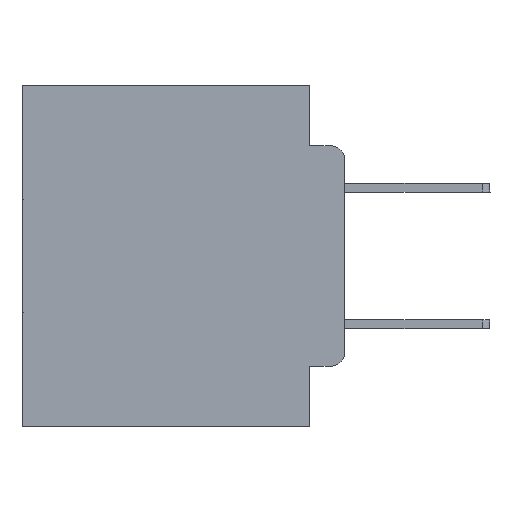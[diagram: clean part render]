
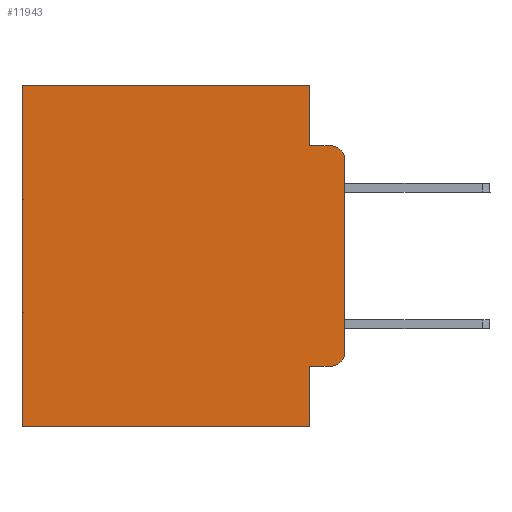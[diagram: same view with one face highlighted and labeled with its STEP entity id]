
A CAD part, left-side view. The second image highlights one B-rep face of the part: STEP entity #11943.
In plain terms, the highlighted planar face has unit normal (-1, 0, 0).
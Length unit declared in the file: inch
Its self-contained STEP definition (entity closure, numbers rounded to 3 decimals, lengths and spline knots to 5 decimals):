
#215 = VERTEX_POINT ( 'NONE', #12271 ) ;
#527 = DIRECTION ( 'NONE',  ( -1., 0., 0. ) ) ;
#592 = VECTOR ( 'NONE', #7287, 39.37008 ) ;
#806 = PLANE ( 'NONE',  #26116 ) ;
#974 = VECTOR ( 'NONE', #10853, 39.37008 ) ;
#2028 = EDGE_CURVE ( 'NONE', #20174, #215, #22887, .T. ) ;
#2127 = VERTEX_POINT ( 'NONE', #13937 ) ;
#3052 = CARTESIAN_POINT ( 'NONE',  ( 0.298, 0.051, 0. ) ) ;
#3873 = EDGE_CURVE ( 'NONE', #20174, #5338, #8511, .T. ) ;
#3918 = VECTOR ( 'NONE', #6177, 39.37008 ) ;
#4004 = CIRCLE ( 'NONE', #19511, 0.02 ) ;
#4091 = VERTEX_POINT ( 'NONE', #21742 ) ;
#4457 = VERTEX_POINT ( 'NONE', #24705 ) ;
#5199 = CARTESIAN_POINT ( 'NONE',  ( 0.298, 0., 0. ) ) ;
#5338 = VERTEX_POINT ( 'NONE', #29000 ) ;
#5693 = DIRECTION ( 'NONE',  ( 0., 0., -1. ) ) ;
#5732 = ORIENTED_EDGE ( 'NONE', *, *, #3873, .F. ) ;
#5999 = LINE ( 'NONE', #8336, #18496 ) ;
#6177 = DIRECTION ( 'NONE',  ( 0., 0., -1. ) ) ;
#6670 = VECTOR ( 'NONE', #21443, 39.37008 ) ;
#7141 = CARTESIAN_POINT ( 'NONE',  ( 0.298, 0.051, -0.4115 ) ) ;
#7287 = DIRECTION ( 'NONE',  ( 0., -1., 0. ) ) ;
#7896 = LINE ( 'NONE', #27117, #17403 ) ;
#8109 = CARTESIAN_POINT ( 'NONE',  ( 0.298, 0.051, -0.0885 ) ) ;
#8336 = CARTESIAN_POINT ( 'NONE',  ( 0.298, 0., -0.5 ) ) ;
#8511 = LINE ( 'NONE', #3052, #3918 ) ;
#8610 = EDGE_CURVE ( 'NONE', #11985, #4457, #7896, .T. ) ;
#8725 = EDGE_CURVE ( 'NONE', #215, #26105, #4004, .T. ) ;
#9983 = EDGE_CURVE ( 'NONE', #30833, #4091, #23713, .T. ) ;
#10091 = DIRECTION ( 'NONE',  ( 0., 0., -1. ) ) ;
#10717 = ORIENTED_EDGE ( 'NONE', *, *, #8610, .T. ) ;
#10837 = EDGE_CURVE ( 'NONE', #4457, #23791, #16733, .T. ) ;
#10853 = DIRECTION ( 'NONE',  ( 0., 0., -1. ) ) ;
#11775 = ORIENTED_EDGE ( 'NONE', *, *, #24284, .F. ) ;
#11791 = CARTESIAN_POINT ( 'NONE',  ( 0.298, 0.051, -0.0885 ) ) ;
#11943 = ADVANCED_FACE ( 'NONE', ( #29594 ), #806, .F. ) ;
#11985 = VERTEX_POINT ( 'NONE', #22252 ) ;
#12154 = AXIS2_PLACEMENT_3D ( 'NONE', #27102, #20222, #24773 ) ;
#12271 = CARTESIAN_POINT ( 'NONE',  ( 0.298, 0.02, -0.4115 ) ) ;
#12841 = CARTESIAN_POINT ( 'NONE',  ( 0.298, 0., 0. ) ) ;
#13098 = EDGE_CURVE ( 'NONE', #2127, #4091, #15145, .T. ) ;
#13292 = EDGE_LOOP ( 'NONE', ( #28618, #15705, #30269, #11775, #10717, #14149, #25980, #5732, #19698, #21313 ) ) ;
#13553 = EDGE_CURVE ( 'NONE', #2127, #26105, #17062, .T. ) ;
#13937 = CARTESIAN_POINT ( 'NONE',  ( 0.298, 0., -0.1085 ) ) ;
#14149 = ORIENTED_EDGE ( 'NONE', *, *, #10837, .T. ) ;
#15145 = CIRCLE ( 'NONE', #12154, 0.02 ) ;
#15705 = ORIENTED_EDGE ( 'NONE', *, *, #13098, .T. ) ;
#16733 = LINE ( 'NONE', #21125, #6670 ) ;
#17062 = LINE ( 'NONE', #5199, #30656 ) ;
#17403 = VECTOR ( 'NONE', #24485, 39.37008 ) ;
#18496 = VECTOR ( 'NONE', #27706, 39.37008 ) ;
#19060 = VECTOR ( 'NONE', #20229, 39.37008 ) ;
#19511 = AXIS2_PLACEMENT_3D ( 'NONE', #24177, #527, #10091 ) ;
#19698 = ORIENTED_EDGE ( 'NONE', *, *, #2028, .T. ) ;
#20096 = CARTESIAN_POINT ( 'NONE',  ( 0.298, 0.051, 0. ) ) ;
#20174 = VERTEX_POINT ( 'NONE', #7141 ) ;
#20222 = DIRECTION ( 'NONE',  ( -1., 0., 0. ) ) ;
#20229 = DIRECTION ( 'NONE',  ( 0., -1., 0. ) ) ;
#21125 = CARTESIAN_POINT ( 'NONE',  ( 0.298, 0.473, 0. ) ) ;
#21313 = ORIENTED_EDGE ( 'NONE', *, *, #8725, .T. ) ;
#21443 = DIRECTION ( 'NONE',  ( 0., 0., -1. ) ) ;
#21592 = CARTESIAN_POINT ( 'NONE',  ( 0.298, 0., -0.3915 ) ) ;
#21742 = CARTESIAN_POINT ( 'NONE',  ( 0.298, 0.02, -0.0885 ) ) ;
#22252 = CARTESIAN_POINT ( 'NONE',  ( 0.298, 0.051, 0. ) ) ;
#22887 = LINE ( 'NONE', #29912, #19060 ) ;
#22911 = LINE ( 'NONE', #20096, #974 ) ;
#23713 = LINE ( 'NONE', #11791, #592 ) ;
#23791 = VERTEX_POINT ( 'NONE', #27623 ) ;
#24177 = CARTESIAN_POINT ( 'NONE',  ( 0.298, 0.02, -0.3915 ) ) ;
#24284 = EDGE_CURVE ( 'NONE', #11985, #30833, #22911, .T. ) ;
#24303 = DIRECTION ( 'NONE',  ( 1., 0., 0. ) ) ;
#24432 = DIRECTION ( 'NONE',  ( 0., 0., -1. ) ) ;
#24485 = DIRECTION ( 'NONE',  ( 0., 1., 0. ) ) ;
#24700 = EDGE_CURVE ( 'NONE', #5338, #23791, #5999, .T. ) ;
#24705 = CARTESIAN_POINT ( 'NONE',  ( 0.298, 0.473, 0. ) ) ;
#24773 = DIRECTION ( 'NONE',  ( 0., 0., -1. ) ) ;
#25980 = ORIENTED_EDGE ( 'NONE', *, *, #24700, .F. ) ;
#26105 = VERTEX_POINT ( 'NONE', #21592 ) ;
#26116 = AXIS2_PLACEMENT_3D ( 'NONE', #12841, #24303, #5693 ) ;
#27102 = CARTESIAN_POINT ( 'NONE',  ( 0.298, 0.02, -0.1085 ) ) ;
#27117 = CARTESIAN_POINT ( 'NONE',  ( 0.298, 0., 0. ) ) ;
#27623 = CARTESIAN_POINT ( 'NONE',  ( 0.298, 0.473, -0.5 ) ) ;
#27706 = DIRECTION ( 'NONE',  ( 0., 1., 0. ) ) ;
#28618 = ORIENTED_EDGE ( 'NONE', *, *, #13553, .F. ) ;
#29000 = CARTESIAN_POINT ( 'NONE',  ( 0.298, 0.051, -0.5 ) ) ;
#29594 = FACE_OUTER_BOUND ( 'NONE', #13292, .T. ) ;
#29912 = CARTESIAN_POINT ( 'NONE',  ( 0.298, 0.051, -0.4115 ) ) ;
#30269 = ORIENTED_EDGE ( 'NONE', *, *, #9983, .F. ) ;
#30656 = VECTOR ( 'NONE', #24432, 39.37008 ) ;
#30833 = VERTEX_POINT ( 'NONE', #8109 ) ;
